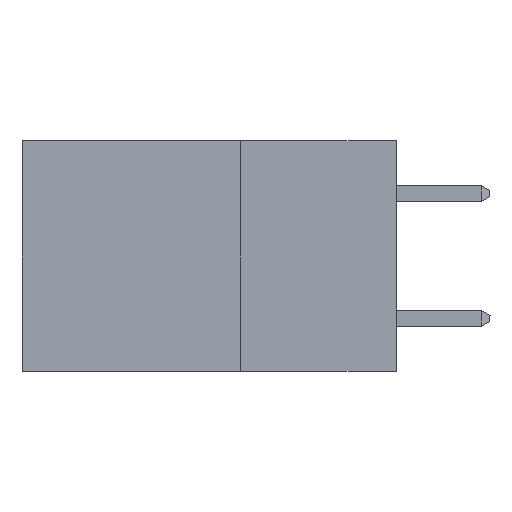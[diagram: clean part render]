
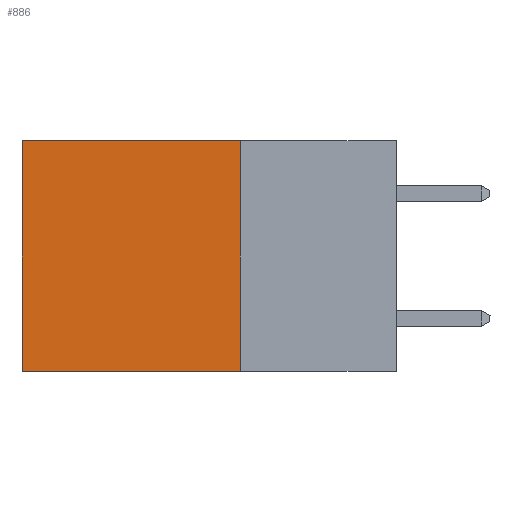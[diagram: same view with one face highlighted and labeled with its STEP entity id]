
A CAD part, left-side view. The second image highlights one B-rep face of the part: STEP entity #886.
In plain terms, the highlighted planar face has unit normal (-1, 0, 0).
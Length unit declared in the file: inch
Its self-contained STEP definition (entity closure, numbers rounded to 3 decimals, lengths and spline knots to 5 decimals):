
#8 = VERTEX_POINT ( 'NONE', #974 ) ;
#260 = VECTOR ( 'NONE', #3433, 39.37008 ) ;
#886 = ADVANCED_FACE ( 'NONE', ( #9548 ), #6986, .F. ) ;
#974 = CARTESIAN_POINT ( 'NONE',  ( 0.2615, 0.25, 0. ) ) ;
#1229 = ORIENTED_EDGE ( 'NONE', *, *, #8608, .T. ) ;
#1742 = VERTEX_POINT ( 'NONE', #10016 ) ;
#1921 = EDGE_CURVE ( 'NONE', #8492, #3620, #12593, .T. ) ;
#2284 = CARTESIAN_POINT ( 'NONE',  ( 0.2615, 0.6, -0.37 ) ) ;
#2892 = LINE ( 'NONE', #6383, #260 ) ;
#2974 = VECTOR ( 'NONE', #12122, 39.37008 ) ;
#3433 = DIRECTION ( 'NONE',  ( 0., 1., 0. ) ) ;
#3560 = ORIENTED_EDGE ( 'NONE', *, *, #12221, .F. ) ;
#3620 = VERTEX_POINT ( 'NONE', #2284 ) ;
#4053 = AXIS2_PLACEMENT_3D ( 'NONE', #4294, #10317, #7001 ) ;
#4294 = CARTESIAN_POINT ( 'NONE',  ( 0.2615, 0.25, -0.37 ) ) ;
#5678 = EDGE_CURVE ( 'NONE', #1742, #3620, #2892, .T. ) ;
#6383 = CARTESIAN_POINT ( 'NONE',  ( 0.2615, 0.25, -0.37 ) ) ;
#6986 = PLANE ( 'NONE',  #4053 ) ;
#7001 = DIRECTION ( 'NONE',  ( 0., 0., -1. ) ) ;
#7180 = CARTESIAN_POINT ( 'NONE',  ( 0.2615, 0.25, 0. ) ) ;
#7664 = CARTESIAN_POINT ( 'NONE',  ( 0.2615, 0.25, -0.37 ) ) ;
#8262 = LINE ( 'NONE', #7180, #2974 ) ;
#8492 = VERTEX_POINT ( 'NONE', #9967 ) ;
#8608 = EDGE_CURVE ( 'NONE', #8, #8492, #8262, .T. ) ;
#8664 = DIRECTION ( 'NONE',  ( 0., 0., -1. ) ) ;
#8757 = ORIENTED_EDGE ( 'NONE', *, *, #1921, .T. ) ;
#8831 = CARTESIAN_POINT ( 'NONE',  ( 0.2615, 0.6, -0.37 ) ) ;
#9352 = DIRECTION ( 'NONE',  ( 0., 0., -1. ) ) ;
#9548 = FACE_OUTER_BOUND ( 'NONE', #12771, .T. ) ;
#9808 = VECTOR ( 'NONE', #8664, 39.37008 ) ;
#9967 = CARTESIAN_POINT ( 'NONE',  ( 0.2615, 0.6, 0. ) ) ;
#9999 = VECTOR ( 'NONE', #9352, 39.37008 ) ;
#10016 = CARTESIAN_POINT ( 'NONE',  ( 0.2615, 0.25, -0.37 ) ) ;
#10317 = DIRECTION ( 'NONE',  ( 1., 0., 0. ) ) ;
#12068 = ORIENTED_EDGE ( 'NONE', *, *, #5678, .F. ) ;
#12122 = DIRECTION ( 'NONE',  ( 0., 1., 0. ) ) ;
#12221 = EDGE_CURVE ( 'NONE', #8, #1742, #12730, .T. ) ;
#12593 = LINE ( 'NONE', #8831, #9999 ) ;
#12730 = LINE ( 'NONE', #7664, #9808 ) ;
#12771 = EDGE_LOOP ( 'NONE', ( #8757, #12068, #3560, #1229 ) ) ;
